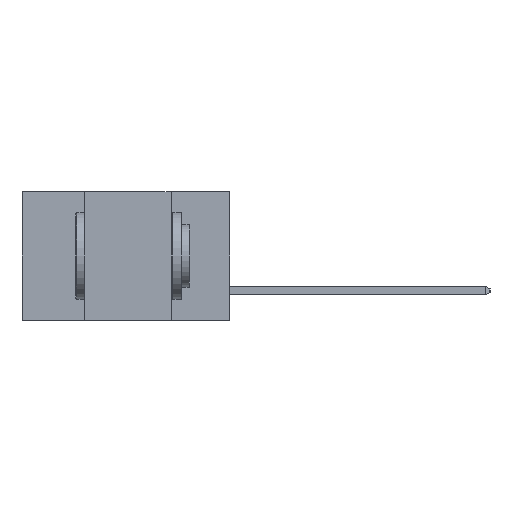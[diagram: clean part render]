
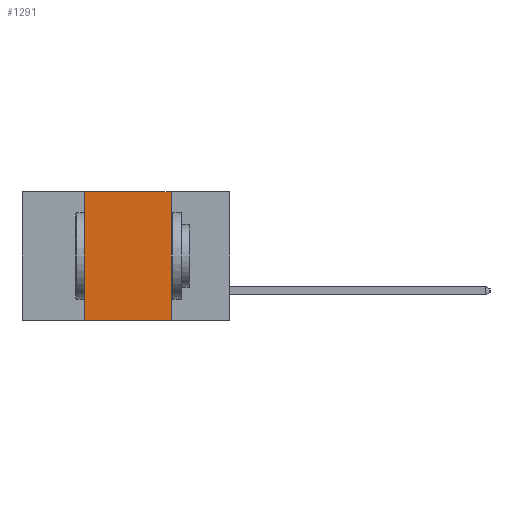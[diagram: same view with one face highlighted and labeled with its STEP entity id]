
A CAD part, left-side view. The second image highlights one B-rep face of the part: STEP entity #1291.
In plain terms, the highlighted planar face has unit normal (-1, 0, 0).
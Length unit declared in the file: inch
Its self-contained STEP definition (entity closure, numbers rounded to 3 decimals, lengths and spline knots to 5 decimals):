
#326 = VECTOR ( 'NONE', #10031, 39.37008 ) ;
#396 = EDGE_CURVE ( 'NONE', #10230, #3821, #789, .T. ) ;
#602 = LINE ( 'NONE', #7721, #3840 ) ;
#789 = LINE ( 'NONE', #12891, #326 ) ;
#1291 = ADVANCED_FACE ( 'NONE', ( #17807 ), #14925, .F. ) ;
#1491 = DIRECTION ( 'NONE',  ( 0., 0., 1. ) ) ;
#1744 = CARTESIAN_POINT ( 'NONE',  ( 0., 0.42, 0. ) ) ;
#1863 = CARTESIAN_POINT ( 'NONE',  ( 0., 0.42, -0.37 ) ) ;
#2669 = ORIENTED_EDGE ( 'NONE', *, *, #396, .T. ) ;
#2774 = AXIS2_PLACEMENT_3D ( 'NONE', #14558, #14869, #14798 ) ;
#2776 = EDGE_CURVE ( 'NONE', #10230, #7797, #12545, .T. ) ;
#3349 = CARTESIAN_POINT ( 'NONE',  ( 0., 0.17, -0.37 ) ) ;
#3560 = DIRECTION ( 'NONE',  ( 0., 0., -1. ) ) ;
#3821 = VERTEX_POINT ( 'NONE', #3349 ) ;
#3840 = VECTOR ( 'NONE', #3560, 39.37008 ) ;
#4348 = ORIENTED_EDGE ( 'NONE', *, *, #13870, .F. ) ;
#4358 = ORIENTED_EDGE ( 'NONE', *, *, #11800, .F. ) ;
#6526 = CARTESIAN_POINT ( 'NONE',  ( 0., 0.42, 0. ) ) ;
#6569 = CARTESIAN_POINT ( 'NONE',  ( 0., 0.6, 0. ) ) ;
#7068 = ORIENTED_EDGE ( 'NONE', *, *, #2776, .F. ) ;
#7721 = CARTESIAN_POINT ( 'NONE',  ( 0., 0.17, 0. ) ) ;
#7797 = VERTEX_POINT ( 'NONE', #6526 ) ;
#7962 = DIRECTION ( 'NONE',  ( 0., -1., 0. ) ) ;
#10031 = DIRECTION ( 'NONE',  ( 0., -1., 0. ) ) ;
#10230 = VERTEX_POINT ( 'NONE', #1863 ) ;
#11431 = CARTESIAN_POINT ( 'NONE',  ( 0., 0.17, 0. ) ) ;
#11800 = EDGE_CURVE ( 'NONE', #7797, #12790, #13204, .T. ) ;
#12545 = LINE ( 'NONE', #1744, #15777 ) ;
#12790 = VERTEX_POINT ( 'NONE', #11431 ) ;
#12891 = CARTESIAN_POINT ( 'NONE',  ( 0., 0.6, -0.37 ) ) ;
#13204 = LINE ( 'NONE', #6569, #13634 ) ;
#13634 = VECTOR ( 'NONE', #7962, 39.37008 ) ;
#13870 = EDGE_CURVE ( 'NONE', #12790, #3821, #602, .T. ) ;
#14558 = CARTESIAN_POINT ( 'NONE',  ( 0., 0.6, 0. ) ) ;
#14588 = EDGE_LOOP ( 'NONE', ( #4348, #4358, #7068, #2669 ) ) ;
#14798 = DIRECTION ( 'NONE',  ( 0., 0., -1. ) ) ;
#14869 = DIRECTION ( 'NONE',  ( 1., 0., 0. ) ) ;
#14925 = PLANE ( 'NONE',  #2774 ) ;
#15777 = VECTOR ( 'NONE', #1491, 39.37008 ) ;
#17807 = FACE_OUTER_BOUND ( 'NONE', #14588, .T. ) ;
